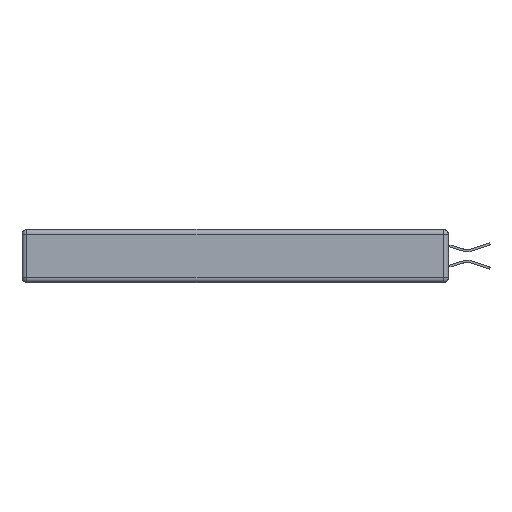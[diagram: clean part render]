
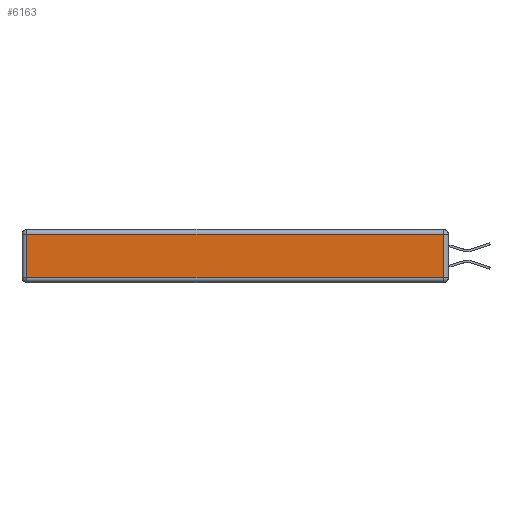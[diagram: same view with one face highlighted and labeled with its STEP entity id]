
A CAD part, left-side view. The second image highlights one B-rep face of the part: STEP entity #6163.
In plain terms, the highlighted planar face has unit normal (-1, 0, 0).
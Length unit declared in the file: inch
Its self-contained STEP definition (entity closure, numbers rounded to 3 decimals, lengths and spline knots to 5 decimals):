
#330 = ORIENTED_EDGE ( 'NONE', *, *, #3802, .T. ) ;
#917 = CARTESIAN_POINT ( 'NONE',  ( 0., 0.03, -0.03 ) ) ;
#928 = DIRECTION ( 'NONE',  ( 0., 0., -1. ) ) ;
#1990 = AXIS2_PLACEMENT_3D ( 'NONE', #2935, #19095, #20954 ) ;
#2049 = LINE ( 'NONE', #4934, #2318 ) ;
#2318 = VECTOR ( 'NONE', #6875, 39.37008 ) ;
#2935 = CARTESIAN_POINT ( 'NONE',  ( 0., 0., -0.343 ) ) ;
#3802 = EDGE_CURVE ( 'NONE', #4570, #16822, #7659, .T. ) ;
#4570 = VERTEX_POINT ( 'NONE', #8654 ) ;
#4934 = CARTESIAN_POINT ( 'NONE',  ( 0., 0., -0.313 ) ) ;
#5113 = EDGE_CURVE ( 'NONE', #19902, #4570, #2049, .T. ) ;
#5147 = VERTEX_POINT ( 'NONE', #10879 ) ;
#6163 = ADVANCED_FACE ( 'NONE', ( #6913 ), #22961, .T. ) ;
#6875 = DIRECTION ( 'NONE',  ( 0., -1., 0. ) ) ;
#6913 = FACE_OUTER_BOUND ( 'NONE', #11207, .T. ) ;
#7659 = LINE ( 'NONE', #14364, #10542 ) ;
#8271 = ORIENTED_EDGE ( 'NONE', *, *, #14190, .T. ) ;
#8654 = CARTESIAN_POINT ( 'NONE',  ( 0., 0.03, -0.313 ) ) ;
#10006 = LINE ( 'NONE', #15800, #19435 ) ;
#10542 = VECTOR ( 'NONE', #16384, 39.37008 ) ;
#10648 = DIRECTION ( 'NONE',  ( 0., 1., 0. ) ) ;
#10879 = CARTESIAN_POINT ( 'NONE',  ( 0., 2.72, -0.03 ) ) ;
#11207 = EDGE_LOOP ( 'NONE', ( #22394, #330, #18877, #8271 ) ) ;
#14190 = EDGE_CURVE ( 'NONE', #5147, #19902, #10006, .T. ) ;
#14279 = CARTESIAN_POINT ( 'NONE',  ( 0., 2.72, -0.313 ) ) ;
#14364 = CARTESIAN_POINT ( 'NONE',  ( 0., 0.03, -0.343 ) ) ;
#15544 = EDGE_CURVE ( 'NONE', #16822, #5147, #21123, .T. ) ;
#15800 = CARTESIAN_POINT ( 'NONE',  ( 0., 2.72, -0.343 ) ) ;
#16384 = DIRECTION ( 'NONE',  ( 0., 0., 1. ) ) ;
#16822 = VERTEX_POINT ( 'NONE', #917 ) ;
#18877 = ORIENTED_EDGE ( 'NONE', *, *, #15544, .T. ) ;
#19095 = DIRECTION ( 'NONE',  ( -1., 0., 0. ) ) ;
#19435 = VECTOR ( 'NONE', #928, 39.37008 ) ;
#19680 = CARTESIAN_POINT ( 'NONE',  ( 0., 2.75, -0.03 ) ) ;
#19902 = VERTEX_POINT ( 'NONE', #14279 ) ;
#20954 = DIRECTION ( 'NONE',  ( 0., 0., 1. ) ) ;
#21123 = LINE ( 'NONE', #19680, #21983 ) ;
#21983 = VECTOR ( 'NONE', #10648, 39.37008 ) ;
#22394 = ORIENTED_EDGE ( 'NONE', *, *, #5113, .T. ) ;
#22961 = PLANE ( 'NONE',  #1990 ) ;
